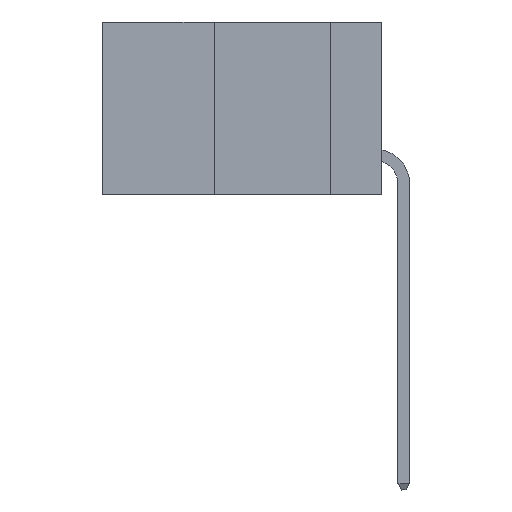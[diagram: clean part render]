
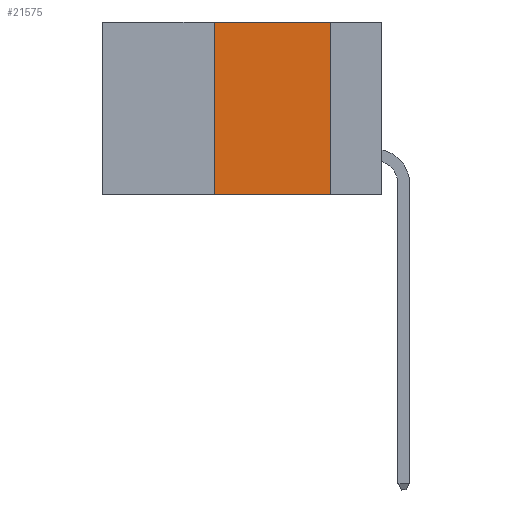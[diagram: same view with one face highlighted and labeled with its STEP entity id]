
A CAD part, left-side view. The second image highlights one B-rep face of the part: STEP entity #21575.
In plain terms, the highlighted planar face has unit normal (-1, 0, 0).
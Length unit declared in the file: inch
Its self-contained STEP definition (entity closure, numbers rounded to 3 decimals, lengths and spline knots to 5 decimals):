
#251 = EDGE_CURVE ( 'NONE', #4062, #8745, #12946, .T. ) ;
#667 = DIRECTION ( 'NONE',  ( 1., 0., 0. ) ) ;
#1207 = CARTESIAN_POINT ( 'NONE',  ( 0., 0.11, 0. ) ) ;
#1258 = CARTESIAN_POINT ( 'NONE',  ( 0., 0.11, -0.37 ) ) ;
#1675 = DIRECTION ( 'NONE',  ( 0., 0., -1. ) ) ;
#2579 = ORIENTED_EDGE ( 'NONE', *, *, #23054, .F. ) ;
#3225 = VECTOR ( 'NONE', #16170, 39.37008 ) ;
#4062 = VERTEX_POINT ( 'NONE', #1207 ) ;
#4251 = PLANE ( 'NONE',  #13091 ) ;
#6870 = LINE ( 'NONE', #13948, #8833 ) ;
#7188 = CARTESIAN_POINT ( 'NONE',  ( 0., 0.11, 0. ) ) ;
#7432 = ORIENTED_EDGE ( 'NONE', *, *, #251, .F. ) ;
#8163 = VECTOR ( 'NONE', #1675, 39.37008 ) ;
#8745 = VERTEX_POINT ( 'NONE', #1258 ) ;
#8833 = VECTOR ( 'NONE', #12313, 39.37008 ) ;
#11539 = CARTESIAN_POINT ( 'NONE',  ( 0., 0.36, -0.37 ) ) ;
#11611 = CARTESIAN_POINT ( 'NONE',  ( 0., 0.6, 0. ) ) ;
#12052 = CARTESIAN_POINT ( 'NONE',  ( 0., 0.6, 0. ) ) ;
#12313 = DIRECTION ( 'NONE',  ( 0., 0., 1. ) ) ;
#12569 = DIRECTION ( 'NONE',  ( 0., -1., 0. ) ) ;
#12946 = LINE ( 'NONE', #7188, #8163 ) ;
#13091 = AXIS2_PLACEMENT_3D ( 'NONE', #11611, #667, #16657 ) ;
#13948 = CARTESIAN_POINT ( 'NONE',  ( 0., 0.36, 0. ) ) ;
#14930 = VECTOR ( 'NONE', #12569, 39.37008 ) ;
#15181 = VERTEX_POINT ( 'NONE', #11539 ) ;
#15449 = EDGE_LOOP ( 'NONE', ( #7432, #2579, #19360, #16081 ) ) ;
#16079 = CARTESIAN_POINT ( 'NONE',  ( 0., 0.36, 0. ) ) ;
#16081 = ORIENTED_EDGE ( 'NONE', *, *, #17148, .T. ) ;
#16114 = LINE ( 'NONE', #12052, #3225 ) ;
#16131 = CARTESIAN_POINT ( 'NONE',  ( 0., 0.6, -0.37 ) ) ;
#16170 = DIRECTION ( 'NONE',  ( 0., -1., 0. ) ) ;
#16345 = EDGE_CURVE ( 'NONE', #15181, #22459, #6870, .T. ) ;
#16657 = DIRECTION ( 'NONE',  ( 0., 0., -1. ) ) ;
#17148 = EDGE_CURVE ( 'NONE', #15181, #8745, #22729, .T. ) ;
#19360 = ORIENTED_EDGE ( 'NONE', *, *, #16345, .F. ) ;
#20333 = FACE_OUTER_BOUND ( 'NONE', #15449, .T. ) ;
#21575 = ADVANCED_FACE ( 'NONE', ( #20333 ), #4251, .F. ) ;
#22459 = VERTEX_POINT ( 'NONE', #16079 ) ;
#22729 = LINE ( 'NONE', #16131, #14930 ) ;
#23054 = EDGE_CURVE ( 'NONE', #22459, #4062, #16114, .T. ) ;
